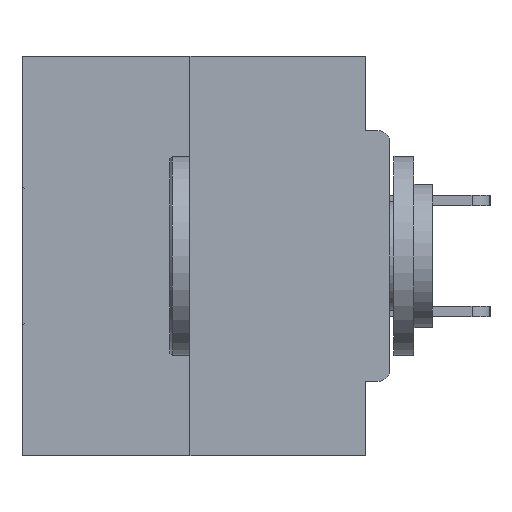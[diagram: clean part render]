
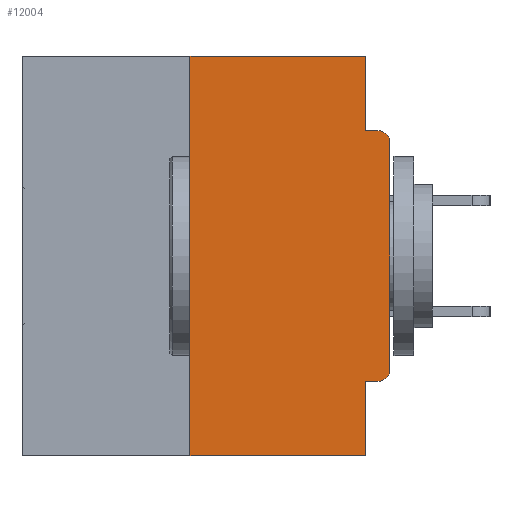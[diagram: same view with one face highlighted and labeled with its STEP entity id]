
A CAD part, left-side view. The second image highlights one B-rep face of the part: STEP entity #12004.
In plain terms, the highlighted planar face has unit normal (-1, 0, 0).
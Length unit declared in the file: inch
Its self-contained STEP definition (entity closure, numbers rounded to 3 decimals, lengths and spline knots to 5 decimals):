
#87 = CARTESIAN_POINT ( 'NONE',  ( 0., 0., -0.1085 ) ) ;
#207 = VERTEX_POINT ( 'NONE', #87 ) ;
#899 = EDGE_CURVE ( 'NONE', #35999, #12670, #28943, .T. ) ;
#1076 = AXIS2_PLACEMENT_3D ( 'NONE', #17949, #18224, #40513 ) ;
#1653 = LINE ( 'NONE', #36872, #28779 ) ;
#2359 = DIRECTION ( 'NONE',  ( 0., 0., 1. ) ) ;
#2640 = EDGE_CURVE ( 'NONE', #12508, #35999, #19319, .T. ) ;
#2828 = CARTESIAN_POINT ( 'NONE',  ( 0., 0., -0.4065 ) ) ;
#3636 = CARTESIAN_POINT ( 'NONE',  ( 0., 0.031, -0.5 ) ) ;
#4296 = CARTESIAN_POINT ( 'NONE',  ( 0., 0.46, -0.5 ) ) ;
#4306 = VECTOR ( 'NONE', #38220, 39.37008 ) ;
#4573 = PLANE ( 'NONE',  #6931 ) ;
#4832 = CARTESIAN_POINT ( 'NONE',  ( 0., 0.031, 0. ) ) ;
#4974 = EDGE_CURVE ( 'NONE', #207, #12670, #35254, .T. ) ;
#6931 = AXIS2_PLACEMENT_3D ( 'NONE', #23941, #39937, #17498 ) ;
#8390 = CARTESIAN_POINT ( 'NONE',  ( 0., 0.25, -0.5 ) ) ;
#8526 = EDGE_CURVE ( 'NONE', #15377, #22682, #22612, .T. ) ;
#8856 = FACE_OUTER_BOUND ( 'NONE', #16211, .T. ) ;
#8875 = ORIENTED_EDGE ( 'NONE', *, *, #21849, .F. ) ;
#10795 = LINE ( 'NONE', #37509, #19288 ) ;
#11340 = CARTESIAN_POINT ( 'NONE',  ( 0., 0., -0.3915 ) ) ;
#11576 = CARTESIAN_POINT ( 'NONE',  ( 0., 0.031, -0.5 ) ) ;
#11751 = ORIENTED_EDGE ( 'NONE', *, *, #2640, .F. ) ;
#12004 = ADVANCED_FACE ( 'NONE', ( #8856 ), #4573, .F. ) ;
#12508 = VERTEX_POINT ( 'NONE', #4832 ) ;
#12670 = VERTEX_POINT ( 'NONE', #19947 ) ;
#13879 = ORIENTED_EDGE ( 'NONE', *, *, #31930, .F. ) ;
#14030 = ORIENTED_EDGE ( 'NONE', *, *, #19182, .T. ) ;
#14740 = VECTOR ( 'NONE', #33214, 39.37008 ) ;
#15377 = VERTEX_POINT ( 'NONE', #39302 ) ;
#15757 = ORIENTED_EDGE ( 'NONE', *, *, #4974, .T. ) ;
#16159 = VERTEX_POINT ( 'NONE', #33306 ) ;
#16211 = EDGE_LOOP ( 'NONE', ( #8875, #24353, #29026, #36054, #13879, #14030, #21830, #15757, #17880, #11751 ) ) ;
#16386 = CIRCLE ( 'NONE', #35328, 0.015 ) ;
#16397 = DIRECTION ( 'NONE',  ( 0., 0., -1. ) ) ;
#16618 = DIRECTION ( 'NONE',  ( 0., -1., 0. ) ) ;
#17498 = DIRECTION ( 'NONE',  ( 0., 0., -1. ) ) ;
#17880 = ORIENTED_EDGE ( 'NONE', *, *, #899, .F. ) ;
#17912 = DIRECTION ( 'NONE',  ( 0., 0., 1. ) ) ;
#17949 = CARTESIAN_POINT ( 'NONE',  ( 0., 0.015, -0.1085 ) ) ;
#18224 = DIRECTION ( 'NONE',  ( -1., 0., 0. ) ) ;
#18231 = LINE ( 'NONE', #4296, #14740 ) ;
#19182 = EDGE_CURVE ( 'NONE', #16159, #20006, #16386, .T. ) ;
#19288 = VECTOR ( 'NONE', #2359, 39.37008 ) ;
#19319 = LINE ( 'NONE', #35200, #31354 ) ;
#19947 = CARTESIAN_POINT ( 'NONE',  ( 0., 0.015, -0.0935 ) ) ;
#20006 = VERTEX_POINT ( 'NONE', #11340 ) ;
#20477 = EDGE_CURVE ( 'NONE', #20006, #207, #10795, .T. ) ;
#21830 = ORIENTED_EDGE ( 'NONE', *, *, #20477, .T. ) ;
#21849 = EDGE_CURVE ( 'NONE', #35395, #12508, #34148, .T. ) ;
#22612 = LINE ( 'NONE', #11576, #32637 ) ;
#22682 = VERTEX_POINT ( 'NONE', #3636 ) ;
#23941 = CARTESIAN_POINT ( 'NONE',  ( 0., 0.46, 0. ) ) ;
#24353 = ORIENTED_EDGE ( 'NONE', *, *, #40340, .F. ) ;
#25486 = CARTESIAN_POINT ( 'NONE',  ( 0., 0.46, 0. ) ) ;
#25801 = DIRECTION ( 'NONE',  ( 0., 0., -1. ) ) ;
#27500 = EDGE_CURVE ( 'NONE', #31717, #22682, #18231, .T. ) ;
#28579 = DIRECTION ( 'NONE',  ( 0., -1., 0. ) ) ;
#28730 = CARTESIAN_POINT ( 'NONE',  ( 0., 0.25, 0. ) ) ;
#28779 = VECTOR ( 'NONE', #17912, 39.37008 ) ;
#28943 = LINE ( 'NONE', #33009, #30944 ) ;
#29026 = ORIENTED_EDGE ( 'NONE', *, *, #27500, .T. ) ;
#29185 = CARTESIAN_POINT ( 'NONE',  ( 0., 0.015, -0.3915 ) ) ;
#29518 = CARTESIAN_POINT ( 'NONE',  ( 0., 0.031, -0.0935 ) ) ;
#30944 = VECTOR ( 'NONE', #16618, 39.37008 ) ;
#31354 = VECTOR ( 'NONE', #25801, 39.37008 ) ;
#31717 = VERTEX_POINT ( 'NONE', #8390 ) ;
#31930 = EDGE_CURVE ( 'NONE', #16159, #15377, #34449, .T. ) ;
#32637 = VECTOR ( 'NONE', #33853, 39.37008 ) ;
#33009 = CARTESIAN_POINT ( 'NONE',  ( 0., 0., -0.0935 ) ) ;
#33214 = DIRECTION ( 'NONE',  ( 0., -1., 0. ) ) ;
#33306 = CARTESIAN_POINT ( 'NONE',  ( 0., 0.015, -0.4065 ) ) ;
#33853 = DIRECTION ( 'NONE',  ( 0., 0., -1. ) ) ;
#34148 = LINE ( 'NONE', #25486, #40673 ) ;
#34449 = LINE ( 'NONE', #2828, #4306 ) ;
#35200 = CARTESIAN_POINT ( 'NONE',  ( 0., 0.031, 0. ) ) ;
#35254 = CIRCLE ( 'NONE', #1076, 0.015 ) ;
#35328 = AXIS2_PLACEMENT_3D ( 'NONE', #29185, #35645, #16397 ) ;
#35395 = VERTEX_POINT ( 'NONE', #28730 ) ;
#35645 = DIRECTION ( 'NONE',  ( -1., 0., 0. ) ) ;
#35999 = VERTEX_POINT ( 'NONE', #29518 ) ;
#36054 = ORIENTED_EDGE ( 'NONE', *, *, #8526, .F. ) ;
#36872 = CARTESIAN_POINT ( 'NONE',  ( 0., 0.25, 0. ) ) ;
#37509 = CARTESIAN_POINT ( 'NONE',  ( 0., 0., 0. ) ) ;
#38220 = DIRECTION ( 'NONE',  ( 0., 1., 0. ) ) ;
#39302 = CARTESIAN_POINT ( 'NONE',  ( 0., 0.031, -0.4065 ) ) ;
#39937 = DIRECTION ( 'NONE',  ( 1., 0., 0. ) ) ;
#40340 = EDGE_CURVE ( 'NONE', #31717, #35395, #1653, .T. ) ;
#40513 = DIRECTION ( 'NONE',  ( 0., 0., -1. ) ) ;
#40673 = VECTOR ( 'NONE', #28579, 39.37008 ) ;
